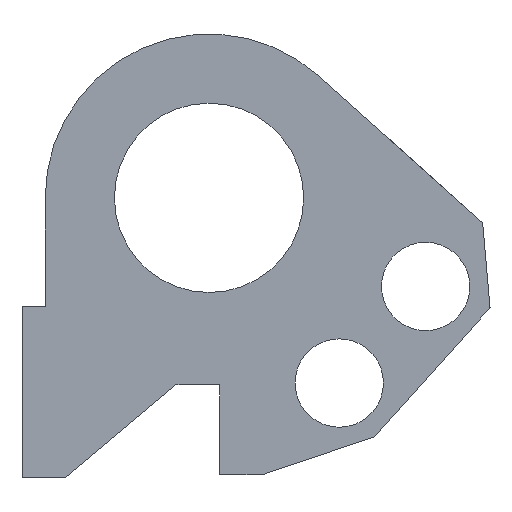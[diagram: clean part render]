
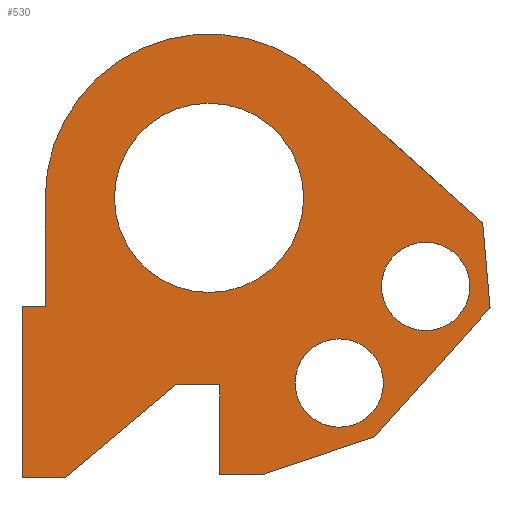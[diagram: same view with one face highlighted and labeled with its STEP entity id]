
A CAD part, left-side view. The second image highlights one B-rep face of the part: STEP entity #530.
In plain terms, the highlighted planar face has unit normal (-1, 0, 0).
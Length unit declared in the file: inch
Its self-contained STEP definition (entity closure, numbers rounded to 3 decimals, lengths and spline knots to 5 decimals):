
#25=FACE_BOUND('',#68,.T.);
#26=FACE_BOUND('',#69,.T.);
#27=FACE_BOUND('',#70,.T.);
#37=FACE_OUTER_BOUND('',#67,.T.);
#67=EDGE_LOOP('',(#393,#394,#395,#396,#397,#398,#399,#400,#401,#402,#403,
#404,#405));
#68=EDGE_LOOP('',(#406));
#69=EDGE_LOOP('',(#407));
#70=EDGE_LOOP('',(#408));
#96=CIRCLE('',#576,0.219);
#97=CIRCLE('',#577,0.1265);
#98=CIRCLE('',#578,0.05906);
#99=CIRCLE('',#579,0.05906);
#119=LINE('',#788,#180);
#122=LINE('',#793,#183);
#124=LINE('',#797,#185);
#126=LINE('',#801,#187);
#128=LINE('',#805,#189);
#130=LINE('',#809,#191);
#131=LINE('',#813,#192);
#132=LINE('',#815,#193);
#133=LINE('',#816,#194);
#134=LINE('',#818,#195);
#135=LINE('',#822,#196);
#136=LINE('',#823,#197);
#180=VECTOR('',#632,0.3937);
#183=VECTOR('',#637,0.3937);
#185=VECTOR('',#641,0.3937);
#187=VECTOR('',#645,0.3937);
#189=VECTOR('',#649,0.3937);
#191=VECTOR('',#653,0.3937);
#192=VECTOR('',#656,0.3937);
#193=VECTOR('',#657,0.3937);
#194=VECTOR('',#658,0.3937);
#195=VECTOR('',#659,0.3937);
#196=VECTOR('',#662,0.3937);
#197=VECTOR('',#663,0.3937);
#244=VERTEX_POINT('',#785);
#245=VERTEX_POINT('',#787);
#246=VERTEX_POINT('',#791);
#247=VERTEX_POINT('',#795);
#248=VERTEX_POINT('',#799);
#249=VERTEX_POINT('',#803);
#250=VERTEX_POINT('',#807);
#251=VERTEX_POINT('',#811);
#252=VERTEX_POINT('',#812);
#253=VERTEX_POINT('',#814);
#254=VERTEX_POINT('',#817);
#255=VERTEX_POINT('',#819);
#256=VERTEX_POINT('',#821);
#257=VERTEX_POINT('',#824);
#258=VERTEX_POINT('',#826);
#259=VERTEX_POINT('',#828);
#295=EDGE_CURVE('',#244,#245,#119,.T.);
#298=EDGE_CURVE('',#246,#244,#122,.T.);
#300=EDGE_CURVE('',#247,#246,#124,.T.);
#302=EDGE_CURVE('',#248,#247,#126,.T.);
#304=EDGE_CURVE('',#249,#248,#128,.T.);
#306=EDGE_CURVE('',#250,#249,#130,.T.);
#307=EDGE_CURVE('',#251,#252,#131,.T.);
#308=EDGE_CURVE('',#253,#251,#132,.T.);
#309=EDGE_CURVE('',#245,#253,#133,.T.);
#310=EDGE_CURVE('',#254,#250,#134,.T.);
#311=EDGE_CURVE('',#255,#254,#96,.T.);
#312=EDGE_CURVE('',#256,#255,#135,.T.);
#313=EDGE_CURVE('',#252,#256,#136,.T.);
#314=EDGE_CURVE('',#257,#257,#97,.T.);
#315=EDGE_CURVE('',#258,#258,#98,.T.);
#316=EDGE_CURVE('',#259,#259,#99,.T.);
#393=ORIENTED_EDGE('',*,*,#307,.F.);
#394=ORIENTED_EDGE('',*,*,#308,.F.);
#395=ORIENTED_EDGE('',*,*,#309,.F.);
#396=ORIENTED_EDGE('',*,*,#295,.F.);
#397=ORIENTED_EDGE('',*,*,#298,.F.);
#398=ORIENTED_EDGE('',*,*,#300,.F.);
#399=ORIENTED_EDGE('',*,*,#302,.F.);
#400=ORIENTED_EDGE('',*,*,#304,.F.);
#401=ORIENTED_EDGE('',*,*,#306,.F.);
#402=ORIENTED_EDGE('',*,*,#310,.F.);
#403=ORIENTED_EDGE('',*,*,#311,.F.);
#404=ORIENTED_EDGE('',*,*,#312,.F.);
#405=ORIENTED_EDGE('',*,*,#313,.F.);
#406=ORIENTED_EDGE('',*,*,#314,.F.);
#407=ORIENTED_EDGE('',*,*,#315,.F.);
#408=ORIENTED_EDGE('',*,*,#316,.F.);
#510=PLANE('',#575);
#530=ADVANCED_FACE('',(#37,#25,#26,#27),#510,.T.);
#575=AXIS2_PLACEMENT_3D('',#810,#654,#655);
#576=AXIS2_PLACEMENT_3D('',#820,#660,#661);
#577=AXIS2_PLACEMENT_3D('',#825,#664,#665);
#578=AXIS2_PLACEMENT_3D('',#827,#666,#667);
#579=AXIS2_PLACEMENT_3D('',#829,#668,#669);
#632=DIRECTION('',(0.,1.,0.));
#637=DIRECTION('',(0.,0.,1.));
#641=DIRECTION('',(0.,1.,0.));
#645=DIRECTION('',(0.,0.948,-0.32));
#649=DIRECTION('',(0.,0.667,-0.745));
#653=DIRECTION('',(0.,-0.086,-0.996));
#654=DIRECTION('center_axis',(-1.,0.,0.));
#655=DIRECTION('ref_axis',(0.,0.,1.));
#656=DIRECTION('',(0.,0.,1.));
#657=DIRECTION('',(0.,1.,0.));
#658=DIRECTION('',(0.,0.766,-0.643));
#659=DIRECTION('',(0.,-0.745,-0.667));
#660=DIRECTION('center_axis',(1.,0.,0.));
#661=DIRECTION('ref_axis',(0.,0.,1.));
#662=DIRECTION('',(0.,0.,1.));
#663=DIRECTION('',(0.,-1.,0.));
#664=DIRECTION('center_axis',(-1.,0.,0.));
#665=DIRECTION('ref_axis',(0.,0.,1.));
#666=DIRECTION('center_axis',(-1.,0.,0.));
#667=DIRECTION('ref_axis',(0.,0.,1.));
#668=DIRECTION('center_axis',(-1.,0.,0.));
#669=DIRECTION('ref_axis',(0.,0.,1.));
#785=CARTESIAN_POINT('',(-0.465,-0.264,3.015));
#787=CARTESIAN_POINT('',(-0.465,-0.20579,3.015));
#788=CARTESIAN_POINT('',(-0.465,-0.28837,3.015));
#791=CARTESIAN_POINT('',(-0.465,-0.264,2.895));
#793=CARTESIAN_POINT('',(-0.465,-0.264,3.01197));
#795=CARTESIAN_POINT('',(-0.465,-0.32114,2.895));
#797=CARTESIAN_POINT('',(-0.465,-0.31694,2.895));
#799=CARTESIAN_POINT('',(-0.465,-0.47136,2.94569));
#801=CARTESIAN_POINT('',(-0.465,-0.42792,2.93103));
#803=CARTESIAN_POINT('',(-0.465,-0.6255,3.11788));
#805=CARTESIAN_POINT('',(-0.465,-0.55869,3.04324));
#807=CARTESIAN_POINT('',(-0.465,-0.61566,3.23161));
#809=CARTESIAN_POINT('',(-0.465,-0.61894,3.19367));
#810=CARTESIAN_POINT('Origin',(-0.465,-0.31275,3.12894));
#811=CARTESIAN_POINT('',(-0.465,0.,2.89116));
#812=CARTESIAN_POINT('',(-0.465,0.,3.12));
#813=CARTESIAN_POINT('',(-0.465,0.,3.07197));
#814=CARTESIAN_POINT('',(-0.465,-0.0582,2.89116));
#815=CARTESIAN_POINT('',(-0.465,-0.15637,2.89116));
#816=CARTESIAN_POINT('',(-0.465,-0.1984,3.0088));
#817=CARTESIAN_POINT('',(-0.465,-0.39606,3.42818));
#818=CARTESIAN_POINT('',(-0.465,-0.48376,3.34968));
#819=CARTESIAN_POINT('',(-0.465,-0.031,3.265));
#820=CARTESIAN_POINT('Origin',(-0.465,-0.25,3.265));
#821=CARTESIAN_POINT('',(-0.465,-0.031,3.12));
#822=CARTESIAN_POINT('',(-0.465,-0.031,3.12447));
#823=CARTESIAN_POINT('',(-0.465,-0.15637,3.12));
#824=CARTESIAN_POINT('',(-0.465,-0.25,3.1385));
#825=CARTESIAN_POINT('Origin',(-0.465,-0.25,3.265));
#826=CARTESIAN_POINT('',(-0.465,-0.424,2.95844));
#827=CARTESIAN_POINT('Origin',(-0.465,-0.424,3.0175));
#828=CARTESIAN_POINT('',(-0.465,-0.53952,3.0875));
#829=CARTESIAN_POINT('Origin',(-0.465,-0.53952,3.14656));
